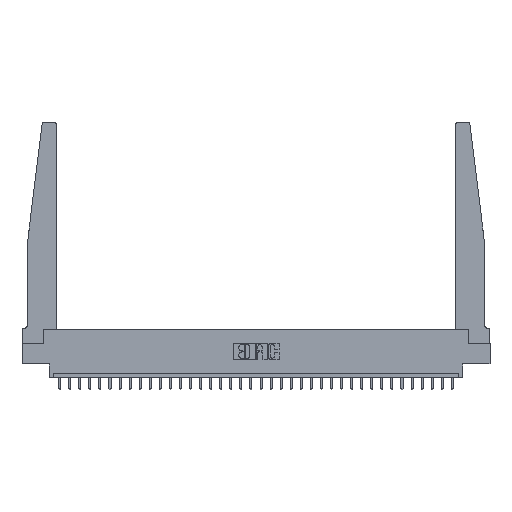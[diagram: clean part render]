
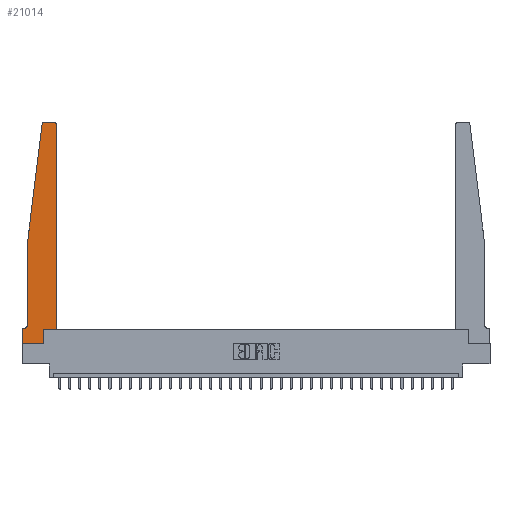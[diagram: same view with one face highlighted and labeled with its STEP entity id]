
A CAD part, top view. The second image highlights one B-rep face of the part: STEP entity #21014.
In plain terms, the highlighted planar face has unit normal (0, 0, 1).
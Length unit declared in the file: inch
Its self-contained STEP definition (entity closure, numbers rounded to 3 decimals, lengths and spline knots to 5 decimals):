
#10 = EDGE_CURVE ( 'NONE', #10677, #27135, #21231, .T. ) ;
#242 = ORIENTED_EDGE ( 'NONE', *, *, #16395, .T. ) ;
#292 = CARTESIAN_POINT ( 'NONE',  ( 0.2605, 0.18, 0.37 ) ) ;
#609 = EDGE_CURVE ( 'NONE', #26453, #10487, #24120, .T. ) ;
#1237 = DIRECTION ( 'NONE',  ( 1., 0., 0. ) ) ;
#1268 = CARTESIAN_POINT ( 'NONE',  ( 0.425, 2.72, 0.37 ) ) ;
#1341 = LINE ( 'NONE', #22356, #26404 ) ;
#1342 = ORIENTED_EDGE ( 'NONE', *, *, #5078, .T. ) ;
#1421 = CARTESIAN_POINT ( 'NONE',  ( 0.065, 1.25, 0.37 ) ) ;
#2016 = AXIS2_PLACEMENT_3D ( 'NONE', #11749, #16202, #14032 ) ;
#2280 = CARTESIAN_POINT ( 'NONE',  ( 0.395, 2.75, 0.37 ) ) ;
#2460 = VERTEX_POINT ( 'NONE', #25579 ) ;
#2935 = CARTESIAN_POINT ( 'NONE',  ( 0.015, 0.2375, 0.37 ) ) ;
#3020 = VECTOR ( 'NONE', #25995, 39.37008 ) ;
#3262 = DIRECTION ( 'NONE',  ( 0., 0., 1. ) ) ;
#3356 = CARTESIAN_POINT ( 'NONE',  ( 0.065, 1.25, 0.37 ) ) ;
#3701 = VECTOR ( 'NONE', #5768, 39.37008 ) ;
#3808 = LINE ( 'NONE', #10944, #24885 ) ;
#4414 = CARTESIAN_POINT ( 'NONE',  ( 0.015, 0.1875, 0.37 ) ) ;
#4891 = ORIENTED_EDGE ( 'NONE', *, *, #7815, .T. ) ;
#5066 = DIRECTION ( 'NONE',  ( -1., 0., 0. ) ) ;
#5078 = EDGE_CURVE ( 'NONE', #10487, #2460, #5139, .T. ) ;
#5139 = LINE ( 'NONE', #12540, #3701 ) ;
#5286 = DIRECTION ( 'NONE',  ( 1., 0., 0. ) ) ;
#5531 = ORIENTED_EDGE ( 'NONE', *, *, #16564, .T. ) ;
#5768 = DIRECTION ( 'NONE',  ( 0., -1., 0. ) ) ;
#6229 = LINE ( 'NONE', #15791, #13175 ) ;
#6355 = ORIENTED_EDGE ( 'NONE', *, *, #609, .T. ) ;
#6781 = ORIENTED_EDGE ( 'NONE', *, *, #12099, .T. ) ;
#7327 = CARTESIAN_POINT ( 'NONE',  ( 0.395, 2.72, 0.37 ) ) ;
#7432 = DIRECTION ( 'NONE',  ( 0., 0., 1. ) ) ;
#7708 = CARTESIAN_POINT ( 'NONE',  ( 0., 0., 0.37 ) ) ;
#7815 = EDGE_CURVE ( 'NONE', #27135, #26794, #20268, .T. ) ;
#8028 = ORIENTED_EDGE ( 'NONE', *, *, #12344, .T. ) ;
#9354 = VERTEX_POINT ( 'NONE', #15527 ) ;
#9447 = CIRCLE ( 'NONE', #2016, 0.03 ) ;
#10328 = EDGE_CURVE ( 'NONE', #9354, #26453, #9447, .T. ) ;
#10358 = CARTESIAN_POINT ( 'NONE',  ( 0.24675, 2.72367, 0.37 ) ) ;
#10475 = CARTESIAN_POINT ( 'NONE',  ( 0.065, 0.1875, 0.37 ) ) ;
#10487 = VERTEX_POINT ( 'NONE', #3356 ) ;
#10677 = VERTEX_POINT ( 'NONE', #11516 ) ;
#10944 = CARTESIAN_POINT ( 'NONE',  ( 0., 0., 0.37 ) ) ;
#11516 = CARTESIAN_POINT ( 'NONE',  ( 0.425, 0.18, 0.37 ) ) ;
#11749 = CARTESIAN_POINT ( 'NONE',  ( 0.27653, 2.72, 0.37 ) ) ;
#12099 = EDGE_CURVE ( 'NONE', #26338, #10677, #1341, .T. ) ;
#12344 = EDGE_CURVE ( 'NONE', #2460, #24340, #14738, .T. ) ;
#12540 = CARTESIAN_POINT ( 'NONE',  ( 0.065, 1.25, 0.37 ) ) ;
#12701 = FACE_OUTER_BOUND ( 'NONE', #18153, .T. ) ;
#13175 = VECTOR ( 'NONE', #17930, 39.37008 ) ;
#13420 = VECTOR ( 'NONE', #20309, 39.37008 ) ;
#13915 = LINE ( 'NONE', #7708, #3020 ) ;
#14032 = DIRECTION ( 'NONE',  ( 1., 0., 0. ) ) ;
#14738 = CIRCLE ( 'NONE', #19977, 0.05 ) ;
#14848 = PLANE ( 'NONE',  #23419 ) ;
#15073 = LINE ( 'NONE', #10475, #18728 ) ;
#15197 = CARTESIAN_POINT ( 'NONE',  ( 0.2605, 0., 0.37 ) ) ;
#15527 = CARTESIAN_POINT ( 'NONE',  ( 0.27653, 2.75, 0.37 ) ) ;
#15791 = CARTESIAN_POINT ( 'NONE',  ( 0.2605, 0.18, 0.37 ) ) ;
#16202 = DIRECTION ( 'NONE',  ( 0., 0., 1. ) ) ;
#16229 = CARTESIAN_POINT ( 'NONE',  ( 0., 0.1875, 0.37 ) ) ;
#16395 = EDGE_CURVE ( 'NONE', #24340, #26759, #15073, .T. ) ;
#16408 = ORIENTED_EDGE ( 'NONE', *, *, #25738, .T. ) ;
#16564 = EDGE_CURVE ( 'NONE', #26541, #20083, #3808, .T. ) ;
#16900 = VECTOR ( 'NONE', #22842, 39.37008 ) ;
#17824 = DIRECTION ( 'NONE',  ( 1., 0., 0. ) ) ;
#17930 = DIRECTION ( 'NONE',  ( 0., 1., 0. ) ) ;
#18153 = EDGE_LOOP ( 'NONE', ( #28844, #19036, #6355, #1342, #8028, #242, #16408, #5531, #29962, #6781, #26713, #4891 ) ) ;
#18728 = VECTOR ( 'NONE', #24736, 39.37008 ) ;
#19036 = ORIENTED_EDGE ( 'NONE', *, *, #10328, .T. ) ;
#19977 = AXIS2_PLACEMENT_3D ( 'NONE', #2935, #28118, #5066 ) ;
#20004 = CARTESIAN_POINT ( 'NONE',  ( 0., 0., 0.37 ) ) ;
#20023 = DIRECTION ( 'NONE',  ( -0.122, -0.992, 0. ) ) ;
#20083 = VERTEX_POINT ( 'NONE', #15197 ) ;
#20268 = CIRCLE ( 'NONE', #22021, 0.03 ) ;
#20309 = DIRECTION ( 'NONE',  ( -1., 0., 0. ) ) ;
#21014 = ADVANCED_FACE ( 'NONE', ( #12701 ), #14848, .T. ) ;
#21231 = LINE ( 'NONE', #25075, #16900 ) ;
#22014 = CARTESIAN_POINT ( 'NONE',  ( 0., 0.1875, 0.37 ) ) ;
#22021 = AXIS2_PLACEMENT_3D ( 'NONE', #7327, #7432, #5286 ) ;
#22356 = CARTESIAN_POINT ( 'NONE',  ( 0.425, 0.18, 0.37 ) ) ;
#22726 = CARTESIAN_POINT ( 'NONE',  ( 0.25, 2.75, 0.37 ) ) ;
#22842 = DIRECTION ( 'NONE',  ( 0., 1., 0. ) ) ;
#22877 = EDGE_CURVE ( 'NONE', #26794, #9354, #28249, .T. ) ;
#23419 = AXIS2_PLACEMENT_3D ( 'NONE', #22014, #3262, #1237 ) ;
#24120 = LINE ( 'NONE', #1421, #27027 ) ;
#24340 = VERTEX_POINT ( 'NONE', #4414 ) ;
#24736 = DIRECTION ( 'NONE',  ( -1., 0., 0. ) ) ;
#24885 = VECTOR ( 'NONE', #24905, 39.37008 ) ;
#24905 = DIRECTION ( 'NONE',  ( 1., 0., 0. ) ) ;
#25075 = CARTESIAN_POINT ( 'NONE',  ( 0.425, 0.18, 0.37 ) ) ;
#25579 = CARTESIAN_POINT ( 'NONE',  ( 0.065, 0.2375, 0.37 ) ) ;
#25738 = EDGE_CURVE ( 'NONE', #26759, #26541, #13915, .T. ) ;
#25995 = DIRECTION ( 'NONE',  ( 0., -1., 0. ) ) ;
#26338 = VERTEX_POINT ( 'NONE', #292 ) ;
#26404 = VECTOR ( 'NONE', #17824, 39.37008 ) ;
#26453 = VERTEX_POINT ( 'NONE', #10358 ) ;
#26541 = VERTEX_POINT ( 'NONE', #20004 ) ;
#26713 = ORIENTED_EDGE ( 'NONE', *, *, #10, .T. ) ;
#26759 = VERTEX_POINT ( 'NONE', #16229 ) ;
#26794 = VERTEX_POINT ( 'NONE', #2280 ) ;
#27027 = VECTOR ( 'NONE', #20023, 39.37008 ) ;
#27135 = VERTEX_POINT ( 'NONE', #1268 ) ;
#27213 = EDGE_CURVE ( 'NONE', #20083, #26338, #6229, .T. ) ;
#28118 = DIRECTION ( 'NONE',  ( 0., 0., -1. ) ) ;
#28249 = LINE ( 'NONE', #22726, #13420 ) ;
#28844 = ORIENTED_EDGE ( 'NONE', *, *, #22877, .T. ) ;
#29962 = ORIENTED_EDGE ( 'NONE', *, *, #27213, .T. ) ;
